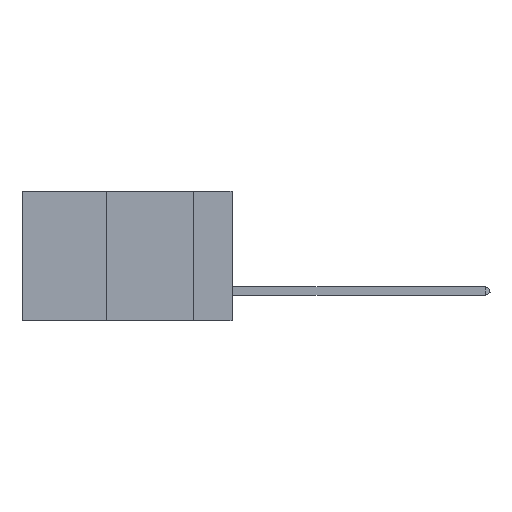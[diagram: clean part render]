
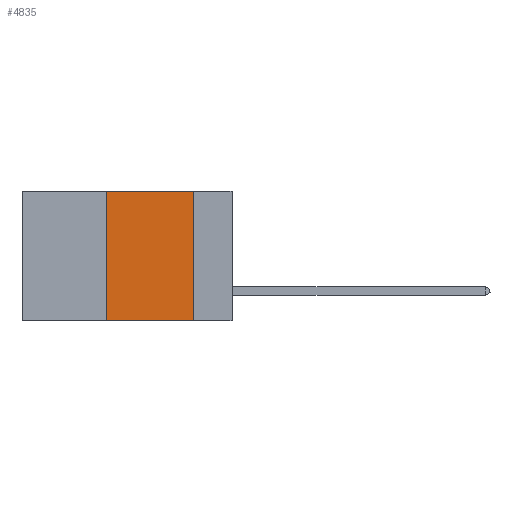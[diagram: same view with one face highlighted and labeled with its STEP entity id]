
A CAD part, left-side view. The second image highlights one B-rep face of the part: STEP entity #4835.
In plain terms, the highlighted planar face has unit normal (-1, 0, 0).
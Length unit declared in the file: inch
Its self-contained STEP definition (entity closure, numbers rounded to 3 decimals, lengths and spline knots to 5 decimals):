
#601 = VECTOR ( 'NONE', #27313, 39.37008 ) ;
#2252 = EDGE_LOOP ( 'NONE', ( #11040, #18799, #5865, #11777 ) ) ;
#3427 = CARTESIAN_POINT ( 'NONE',  ( 0., 0.11, -0.37 ) ) ;
#4835 = ADVANCED_FACE ( 'NONE', ( #10189 ), #13760, .F. ) ;
#5865 = ORIENTED_EDGE ( 'NONE', *, *, #11558, .F. ) ;
#7075 = DIRECTION ( 'NONE',  ( 0., 0., 1. ) ) ;
#8327 = VECTOR ( 'NONE', #22177, 39.37008 ) ;
#9718 = CARTESIAN_POINT ( 'NONE',  ( 0., 0.11, 0. ) ) ;
#10189 = FACE_OUTER_BOUND ( 'NONE', #2252, .T. ) ;
#10845 = VERTEX_POINT ( 'NONE', #24350 ) ;
#10856 = VECTOR ( 'NONE', #7075, 39.37008 ) ;
#11040 = ORIENTED_EDGE ( 'NONE', *, *, #13439, .F. ) ;
#11558 = EDGE_CURVE ( 'NONE', #17621, #10845, #29177, .T. ) ;
#11777 = ORIENTED_EDGE ( 'NONE', *, *, #24978, .T. ) ;
#12167 = CARTESIAN_POINT ( 'NONE',  ( 0., 0.6, 0. ) ) ;
#13374 = LINE ( 'NONE', #14838, #601 ) ;
#13439 = EDGE_CURVE ( 'NONE', #31188, #18434, #23844, .T. ) ;
#13760 = PLANE ( 'NONE',  #31455 ) ;
#14838 = CARTESIAN_POINT ( 'NONE',  ( 0., 0.6, -0.37 ) ) ;
#16909 = VECTOR ( 'NONE', #19934, 39.37008 ) ;
#17621 = VERTEX_POINT ( 'NONE', #31142 ) ;
#18434 = VERTEX_POINT ( 'NONE', #3427 ) ;
#18799 = ORIENTED_EDGE ( 'NONE', *, *, #25511, .F. ) ;
#18886 = DIRECTION ( 'NONE',  ( 0., 0., -1. ) ) ;
#19934 = DIRECTION ( 'NONE',  ( 0., -1., 0. ) ) ;
#22177 = DIRECTION ( 'NONE',  ( 0., 0., -1. ) ) ;
#23844 = LINE ( 'NONE', #9718, #8327 ) ;
#24110 = CARTESIAN_POINT ( 'NONE',  ( 0., 0.6, 0. ) ) ;
#24350 = CARTESIAN_POINT ( 'NONE',  ( 0., 0.36, 0. ) ) ;
#24750 = CARTESIAN_POINT ( 'NONE',  ( 0., 0.11, 0. ) ) ;
#24978 = EDGE_CURVE ( 'NONE', #17621, #18434, #13374, .T. ) ;
#24990 = CARTESIAN_POINT ( 'NONE',  ( 0., 0.36, 0. ) ) ;
#25511 = EDGE_CURVE ( 'NONE', #10845, #31188, #26105, .T. ) ;
#26105 = LINE ( 'NONE', #12167, #16909 ) ;
#26366 = DIRECTION ( 'NONE',  ( 1., 0., 0. ) ) ;
#27313 = DIRECTION ( 'NONE',  ( 0., -1., 0. ) ) ;
#29177 = LINE ( 'NONE', #24990, #10856 ) ;
#31142 = CARTESIAN_POINT ( 'NONE',  ( 0., 0.36, -0.37 ) ) ;
#31188 = VERTEX_POINT ( 'NONE', #24750 ) ;
#31455 = AXIS2_PLACEMENT_3D ( 'NONE', #24110, #26366, #18886 ) ;
